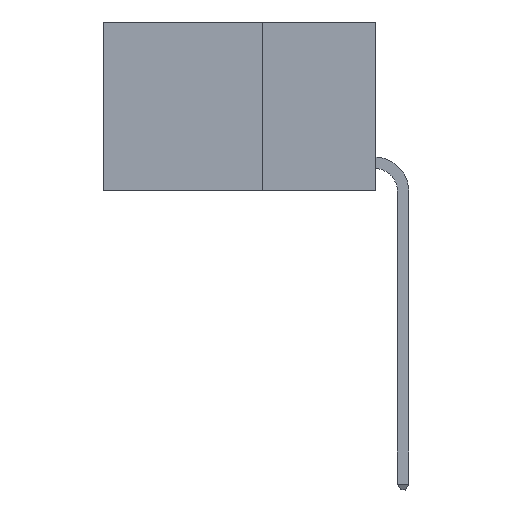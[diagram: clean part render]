
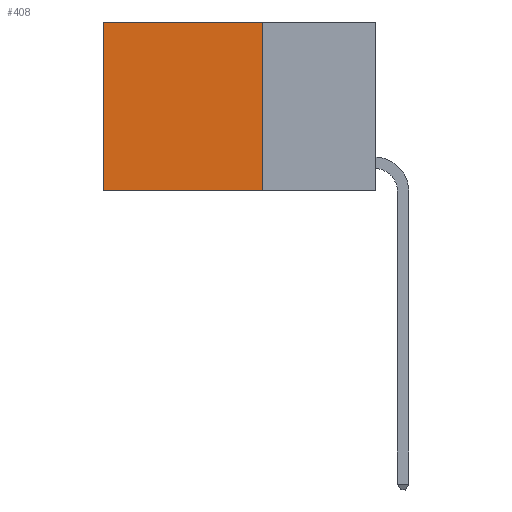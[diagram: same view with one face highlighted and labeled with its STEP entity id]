
A CAD part, left-side view. The second image highlights one B-rep face of the part: STEP entity #408.
In plain terms, the highlighted planar face has unit normal (-1, 0, 0).
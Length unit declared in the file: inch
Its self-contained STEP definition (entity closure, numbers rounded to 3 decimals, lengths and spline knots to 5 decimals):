
#77 = CARTESIAN_POINT ( 'NONE',  ( 0.2625, 0.25, -0.37 ) ) ;
#99 = ORIENTED_EDGE ( 'NONE', *, *, #9187, .T. ) ;
#243 = CARTESIAN_POINT ( 'NONE',  ( 0.2625, 0.6, 0. ) ) ;
#408 = ADVANCED_FACE ( 'NONE', ( #5502 ), #4052, .F. ) ;
#442 = DIRECTION ( 'NONE',  ( 0., 0., -1. ) ) ;
#547 = VERTEX_POINT ( 'NONE', #1153 ) ;
#1010 = ORIENTED_EDGE ( 'NONE', *, *, #9211, .F. ) ;
#1153 = CARTESIAN_POINT ( 'NONE',  ( 0.2625, 0.25, 0. ) ) ;
#1350 = VECTOR ( 'NONE', #442, 39.37008 ) ;
#1629 = EDGE_CURVE ( 'NONE', #547, #6413, #1894, .T. ) ;
#1862 = ORIENTED_EDGE ( 'NONE', *, *, #6099, .F. ) ;
#1894 = LINE ( 'NONE', #5096, #4071 ) ;
#2566 = CARTESIAN_POINT ( 'NONE',  ( 0.2625, 0.25, 0. ) ) ;
#2859 = LINE ( 'NONE', #2566, #6876 ) ;
#3040 = DIRECTION ( 'NONE',  ( 0., 0., -1. ) ) ;
#3384 = DIRECTION ( 'NONE',  ( 0., 0., -1. ) ) ;
#3574 = LINE ( 'NONE', #8666, #1350 ) ;
#4052 = PLANE ( 'NONE',  #5061 ) ;
#4071 = VECTOR ( 'NONE', #5148, 39.37008 ) ;
#4143 = VERTEX_POINT ( 'NONE', #4638 ) ;
#4638 = CARTESIAN_POINT ( 'NONE',  ( 0.2625, 0.6, -0.37 ) ) ;
#5061 = AXIS2_PLACEMENT_3D ( 'NONE', #8554, #8643, #3040 ) ;
#5096 = CARTESIAN_POINT ( 'NONE',  ( 0.2625, 0.25, 0. ) ) ;
#5148 = DIRECTION ( 'NONE',  ( 0., 1., 0. ) ) ;
#5502 = FACE_OUTER_BOUND ( 'NONE', #6504, .T. ) ;
#5717 = VECTOR ( 'NONE', #7883, 39.37008 ) ;
#5964 = LINE ( 'NONE', #10246, #5717 ) ;
#6099 = EDGE_CURVE ( 'NONE', #547, #10325, #2859, .T. ) ;
#6413 = VERTEX_POINT ( 'NONE', #243 ) ;
#6504 = EDGE_LOOP ( 'NONE', ( #99, #1010, #1862, #6920 ) ) ;
#6876 = VECTOR ( 'NONE', #3384, 39.37008 ) ;
#6920 = ORIENTED_EDGE ( 'NONE', *, *, #1629, .T. ) ;
#7883 = DIRECTION ( 'NONE',  ( 0., 1., 0. ) ) ;
#8554 = CARTESIAN_POINT ( 'NONE',  ( 0.2625, 0.25, 0. ) ) ;
#8643 = DIRECTION ( 'NONE',  ( 1., 0., 0. ) ) ;
#8666 = CARTESIAN_POINT ( 'NONE',  ( 0.2625, 0.6, 0. ) ) ;
#9187 = EDGE_CURVE ( 'NONE', #6413, #4143, #3574, .T. ) ;
#9211 = EDGE_CURVE ( 'NONE', #10325, #4143, #5964, .T. ) ;
#10246 = CARTESIAN_POINT ( 'NONE',  ( 0.2625, 0.25, -0.37 ) ) ;
#10325 = VERTEX_POINT ( 'NONE', #77 ) ;
